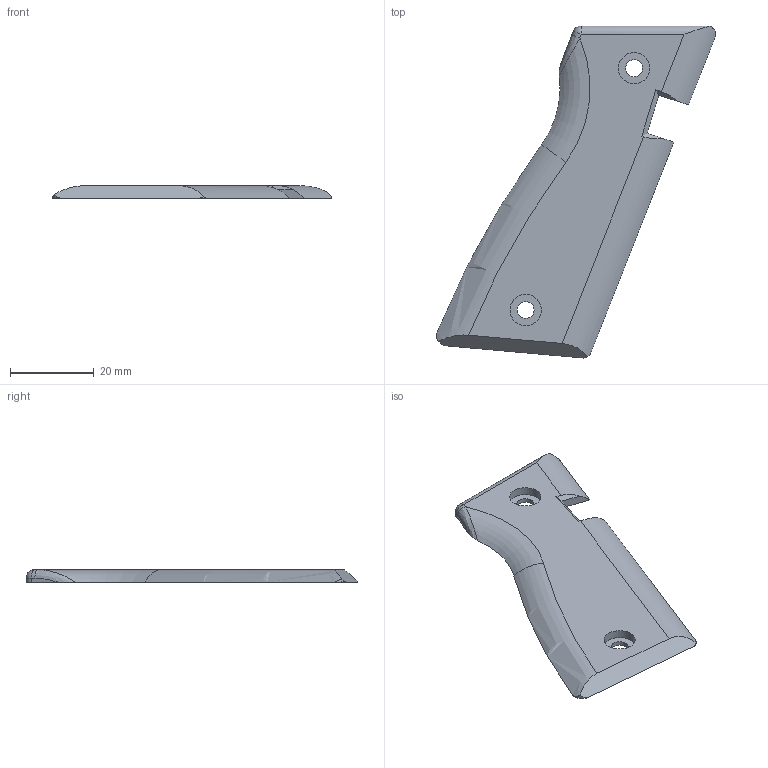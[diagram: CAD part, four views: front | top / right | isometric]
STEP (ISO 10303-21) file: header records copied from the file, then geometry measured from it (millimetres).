
FILE_DESCRIPTION(/* description */ (''),/* implementation_level */ '2;1');
FILE_NAME(/* name */ 'G19Eleven Right Rounded Grip.step',/* time_stamp */ '2022-05-10T10:24:32-06:00',/* author */ (''),/* organization */ (''),/* preprocessor_version */ 'ST-DEVELOPER v18.1',/* originating_system */ 'Autodesk Translation Framework v10.14.0.1471',/* authorisation */ '');
FILE_SCHEMA (('AUTOMOTIVE_DESIGN { 1 0 10303 214 3 1 1 }'));
Length unit declared in the file: millimetre
Products named in the file (1): G1911
Bounding box: 66.53 x 79.14 x 3 mm (x, y, z)
Volume: 6543.4 mm3; surface area: 5644.5 mm2
Topology: 1 solids, 1 shells, 31 faces, 75 edges, 48 vertices
Faces by surface type: plane 14, cylinder 13, torus 2, bspline 1, sphere 1
Full cylindrical faces by diameter (mm): 4 x2, 7.5 x2
Entity records: 1032 total; most frequent: CARTESIAN_POINT 242, DIRECTION 158, ORIENTED_EDGE 150, EDGE_CURVE 75, AXIS2_PLACEMENT_3D 61, VERTEX_POINT 48, EDGE_LOOP 37, LINE 36
